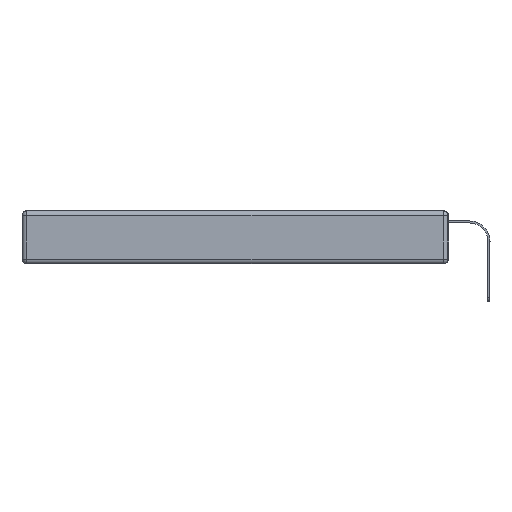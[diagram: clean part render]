
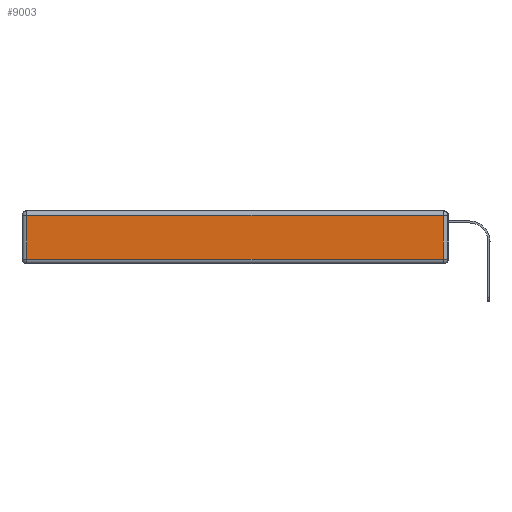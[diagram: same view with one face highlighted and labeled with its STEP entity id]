
A CAD part, left-side view. The second image highlights one B-rep face of the part: STEP entity #9003.
In plain terms, the highlighted planar face has unit normal (-1, 0, 0).
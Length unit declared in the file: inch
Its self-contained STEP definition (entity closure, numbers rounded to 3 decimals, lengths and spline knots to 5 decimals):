
#585 = EDGE_CURVE ( 'NONE', #24134, #9894, #21323, .T. ) ;
#2159 = VERTEX_POINT ( 'NONE', #6228 ) ;
#2625 = ORIENTED_EDGE ( 'NONE', *, *, #585, .T. ) ;
#2906 = ORIENTED_EDGE ( 'NONE', *, *, #25318, .T. ) ;
#3241 = AXIS2_PLACEMENT_3D ( 'NONE', #12125, #13944, #14072 ) ;
#4340 = PLANE ( 'NONE',  #3241 ) ;
#5156 = CARTESIAN_POINT ( 'NONE',  ( 0., 0.03, -0.343 ) ) ;
#6228 = CARTESIAN_POINT ( 'NONE',  ( 0., 0.03, -0.03 ) ) ;
#6685 = VECTOR ( 'NONE', #8930, 39.37008 ) ;
#6964 = CARTESIAN_POINT ( 'NONE',  ( 0., 2.72, -0.343 ) ) ;
#7775 = CARTESIAN_POINT ( 'NONE',  ( 0., 0.03, -0.313 ) ) ;
#8930 = DIRECTION ( 'NONE',  ( 0., 0., -1. ) ) ;
#9003 = ADVANCED_FACE ( 'NONE', ( #24339 ), #4340, .T. ) ;
#9177 = DIRECTION ( 'NONE',  ( 0., 0., 1. ) ) ;
#9357 = CARTESIAN_POINT ( 'NONE',  ( 0., 0., -0.313 ) ) ;
#9894 = VERTEX_POINT ( 'NONE', #7775 ) ;
#11753 = VECTOR ( 'NONE', #9177, 39.37008 ) ;
#11762 = CARTESIAN_POINT ( 'NONE',  ( 0., 2.72, -0.03 ) ) ;
#12125 = CARTESIAN_POINT ( 'NONE',  ( 0., 0., -0.343 ) ) ;
#13004 = VECTOR ( 'NONE', #23626, 39.37008 ) ;
#13944 = DIRECTION ( 'NONE',  ( -1., 0., 0. ) ) ;
#14072 = DIRECTION ( 'NONE',  ( 0., 0., 1. ) ) ;
#14830 = EDGE_CURVE ( 'NONE', #9894, #2159, #15416, .T. ) ;
#14954 = DIRECTION ( 'NONE',  ( 0., -1., 0. ) ) ;
#15416 = LINE ( 'NONE', #5156, #11753 ) ;
#15704 = CARTESIAN_POINT ( 'NONE',  ( 0., 2.75, -0.03 ) ) ;
#16352 = ORIENTED_EDGE ( 'NONE', *, *, #22677, .T. ) ;
#16474 = CARTESIAN_POINT ( 'NONE',  ( 0., 2.72, -0.313 ) ) ;
#18019 = VECTOR ( 'NONE', #14954, 39.37008 ) ;
#19069 = EDGE_LOOP ( 'NONE', ( #2625, #20223, #2906, #16352 ) ) ;
#20223 = ORIENTED_EDGE ( 'NONE', *, *, #14830, .T. ) ;
#21323 = LINE ( 'NONE', #9357, #18019 ) ;
#21934 = LINE ( 'NONE', #15704, #13004 ) ;
#22325 = LINE ( 'NONE', #6964, #6685 ) ;
#22677 = EDGE_CURVE ( 'NONE', #22989, #24134, #22325, .T. ) ;
#22989 = VERTEX_POINT ( 'NONE', #11762 ) ;
#23626 = DIRECTION ( 'NONE',  ( 0., 1., 0. ) ) ;
#24134 = VERTEX_POINT ( 'NONE', #16474 ) ;
#24339 = FACE_OUTER_BOUND ( 'NONE', #19069, .T. ) ;
#25318 = EDGE_CURVE ( 'NONE', #2159, #22989, #21934, .T. ) ;
